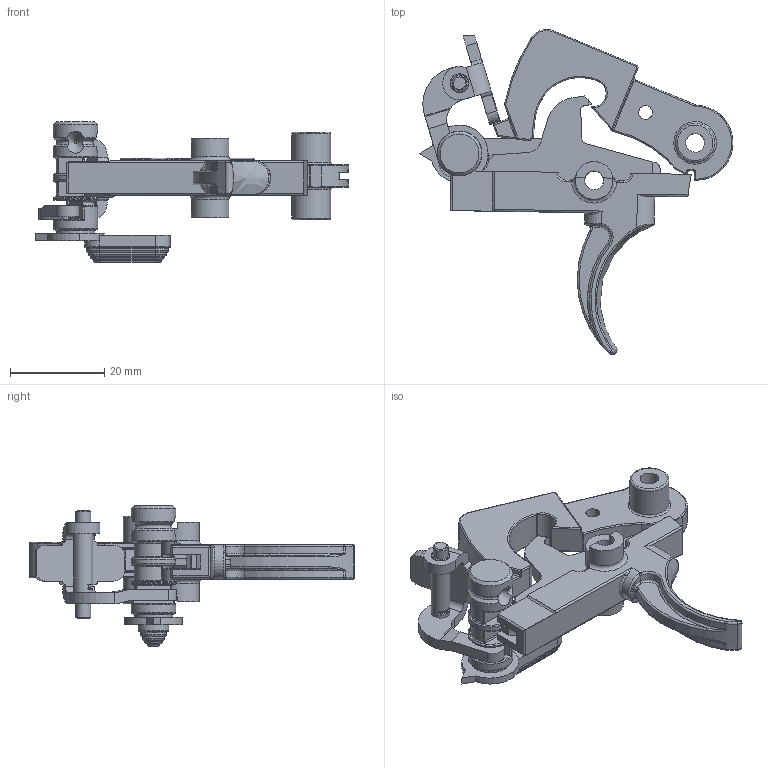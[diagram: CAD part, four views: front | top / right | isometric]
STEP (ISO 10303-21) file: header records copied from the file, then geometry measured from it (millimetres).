
FILE_DESCRIPTION(/* description */ (''),/* implementation_level */ '2;1');
FILE_NAME(/* name */ 'M16 FCG.stp',/* time_stamp */ '2019-01-20T15:26:34-06:00',/* author */ ('johne'),/* organization */ (''),/* preprocessor_version */ 'ST-DEVELOPER v16.13',/* originating_system */ 'Autodesk Inventor 2018',/* authorisation */ '');
FILE_SCHEMA (('AUTOMOTIVE_DESIGN { 1 0 10303 214 3 1 1 }'));
Length unit declared in the file: inch
Products named in the file (8): FA FCG; M16 Disco V2; Auto Sear Pin; Selector M16 V2; Auto Sear Bushing; Auto Sear; Auto Trigger; M16 Hammer V5
Assembly tree (7 placements, depth 2):
  FA FCG
    M16 Disco V2
    Auto Sear Pin
    Selector M16 V2
    Auto Sear Bushing
    Auto Sear
    Auto Trigger
    M16 Hammer V5
Bounding box: 66.54 x 68.94 x 29.74 mm (x, y, z)
Volume: 11661.8 mm3; surface area: 10649.5 mm2
Topology: 8 solids, 8 shells, 573 faces, 1407 edges, 838 vertices
Faces by surface type: cylinder 200, plane 169, torus 97, bspline 70, sphere 25, cone 12
Full cylindrical faces by diameter (mm): 2.946 x1, 3.023 x1, 3.124 x3, 3.188 x1, 3.95 x2, 3.962 x3, 4.013 x2, 4.216 x1, 7.986 x2, 8.255 x1, 8.28 x2, 9.474 x4
Entity records: 25884 total; most frequent: CARTESIAN_POINT 12552, DIRECTION 2808, ORIENTED_EDGE 2664, EDGE_CURVE 1332, AXIS2_PLACEMENT_3D 1122, VERTEX_POINT 823, EDGE_LOOP 643, FACE_OUTER_BOUND 573
